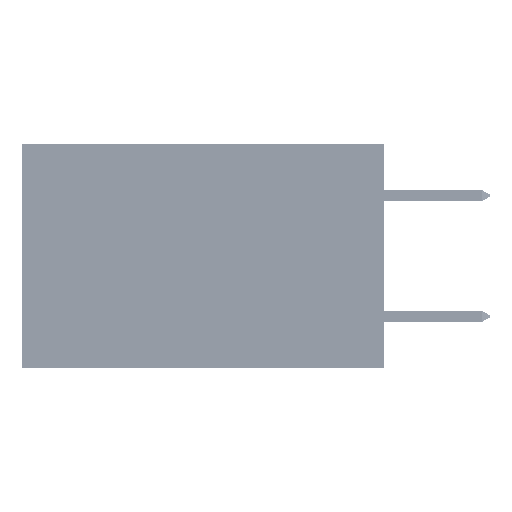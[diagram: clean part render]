
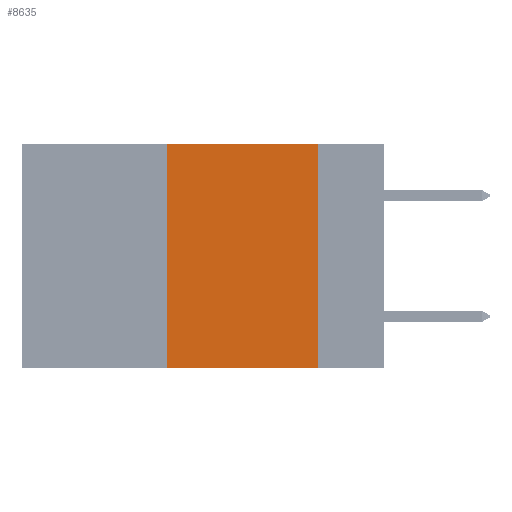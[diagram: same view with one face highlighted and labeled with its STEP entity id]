
A CAD part, left-side view. The second image highlights one B-rep face of the part: STEP entity #8635.
In plain terms, the highlighted planar face has unit normal (-1, 0, 0).
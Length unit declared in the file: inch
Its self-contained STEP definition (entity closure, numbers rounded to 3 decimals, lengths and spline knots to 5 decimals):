
#1479 = CARTESIAN_POINT ( 'NONE',  ( 0., 0.6, -0.37 ) ) ;
#3318 = ORIENTED_EDGE ( 'NONE', *, *, #35409, .F. ) ;
#3526 = VERTEX_POINT ( 'NONE', #31535 ) ;
#3848 = CARTESIAN_POINT ( 'NONE',  ( 0., 0.6, 0. ) ) ;
#5030 = DIRECTION ( 'NONE',  ( 0., -1., 0. ) ) ;
#5598 = FACE_OUTER_BOUND ( 'NONE', #35949, .T. ) ;
#8293 = VECTOR ( 'NONE', #5030, 39.37008 ) ;
#8635 = ADVANCED_FACE ( 'NONE', ( #5598 ), #34750, .F. ) ;
#9309 = AXIS2_PLACEMENT_3D ( 'NONE', #27640, #38245, #17214 ) ;
#13034 = EDGE_CURVE ( 'NONE', #41425, #21572, #34153, .T. ) ;
#16702 = ORIENTED_EDGE ( 'NONE', *, *, #31373, .F. ) ;
#17214 = DIRECTION ( 'NONE',  ( 0., 0., -1. ) ) ;
#21572 = VERTEX_POINT ( 'NONE', #42496 ) ;
#23388 = VECTOR ( 'NONE', #26973, 39.37008 ) ;
#23421 = CARTESIAN_POINT ( 'NONE',  ( 0., 0.11, 0. ) ) ;
#25520 = ORIENTED_EDGE ( 'NONE', *, *, #13034, .T. ) ;
#25802 = LINE ( 'NONE', #36595, #43417 ) ;
#26973 = DIRECTION ( 'NONE',  ( 0., 0., -1. ) ) ;
#27640 = CARTESIAN_POINT ( 'NONE',  ( 0., 0.6, 0. ) ) ;
#31373 = EDGE_CURVE ( 'NONE', #39132, #21572, #41006, .T. ) ;
#31535 = CARTESIAN_POINT ( 'NONE',  ( 0., 0.36, 0. ) ) ;
#31691 = EDGE_CURVE ( 'NONE', #3526, #39132, #38244, .T. ) ;
#31990 = CARTESIAN_POINT ( 'NONE',  ( 0., 0.11, 0. ) ) ;
#34153 = LINE ( 'NONE', #1479, #8293 ) ;
#34750 = PLANE ( 'NONE',  #9309 ) ;
#34906 = ORIENTED_EDGE ( 'NONE', *, *, #31691, .F. ) ;
#35409 = EDGE_CURVE ( 'NONE', #41425, #3526, #25802, .T. ) ;
#35949 = EDGE_LOOP ( 'NONE', ( #16702, #34906, #3318, #25520 ) ) ;
#36595 = CARTESIAN_POINT ( 'NONE',  ( 0., 0.36, 0. ) ) ;
#37157 = VECTOR ( 'NONE', #38954, 39.37008 ) ;
#38244 = LINE ( 'NONE', #3848, #37157 ) ;
#38245 = DIRECTION ( 'NONE',  ( 1., 0., 0. ) ) ;
#38954 = DIRECTION ( 'NONE',  ( 0., -1., 0. ) ) ;
#39132 = VERTEX_POINT ( 'NONE', #31990 ) ;
#40879 = CARTESIAN_POINT ( 'NONE',  ( 0., 0.36, -0.37 ) ) ;
#41006 = LINE ( 'NONE', #23421, #23388 ) ;
#41425 = VERTEX_POINT ( 'NONE', #40879 ) ;
#42496 = CARTESIAN_POINT ( 'NONE',  ( 0., 0.11, -0.37 ) ) ;
#43417 = VECTOR ( 'NONE', #43611, 39.37008 ) ;
#43611 = DIRECTION ( 'NONE',  ( 0., 0., 1. ) ) ;
